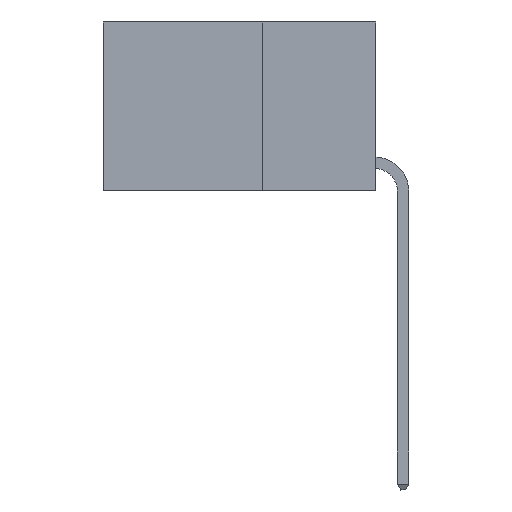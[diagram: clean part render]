
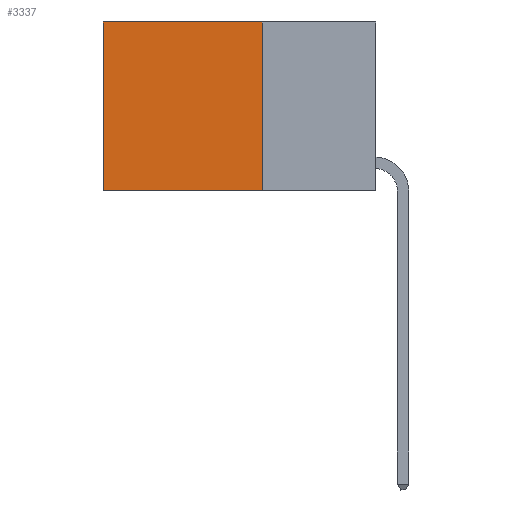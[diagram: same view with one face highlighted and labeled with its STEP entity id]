
A CAD part, left-side view. The second image highlights one B-rep face of the part: STEP entity #3337.
In plain terms, the highlighted planar face has unit normal (-1, 0, 0).
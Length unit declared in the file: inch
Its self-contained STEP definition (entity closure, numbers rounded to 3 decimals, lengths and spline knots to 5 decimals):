
#64 = CARTESIAN_POINT ( 'NONE',  ( 0.2625, 0.25, -0.37 ) ) ;
#413 = CARTESIAN_POINT ( 'NONE',  ( 0.2625, 0.6, 0. ) ) ;
#586 = CARTESIAN_POINT ( 'NONE',  ( 0.2625, 0.25, -0.37 ) ) ;
#1047 = AXIS2_PLACEMENT_3D ( 'NONE', #17012, #5316, #1689 ) ;
#1689 = DIRECTION ( 'NONE',  ( 0., 0., -1. ) ) ;
#3337 = ADVANCED_FACE ( 'NONE', ( #10134 ), #10241, .F. ) ;
#5316 = DIRECTION ( 'NONE',  ( 1., 0., 0. ) ) ;
#6028 = VECTOR ( 'NONE', #9191, 39.37008 ) ;
#6531 = VERTEX_POINT ( 'NONE', #8507 ) ;
#6735 = EDGE_CURVE ( 'NONE', #6531, #14203, #7397, .T. ) ;
#7397 = LINE ( 'NONE', #13955, #15891 ) ;
#8507 = CARTESIAN_POINT ( 'NONE',  ( 0.2625, 0.25, 0. ) ) ;
#8695 = ORIENTED_EDGE ( 'NONE', *, *, #10367, .T. ) ;
#9191 = DIRECTION ( 'NONE',  ( 0., 0., -1. ) ) ;
#9387 = VERTEX_POINT ( 'NONE', #586 ) ;
#9735 = LINE ( 'NONE', #11099, #17660 ) ;
#10134 = FACE_OUTER_BOUND ( 'NONE', #20794, .T. ) ;
#10232 = ORIENTED_EDGE ( 'NONE', *, *, #16934, .F. ) ;
#10241 = PLANE ( 'NONE',  #1047 ) ;
#10367 = EDGE_CURVE ( 'NONE', #14203, #20745, #9735, .T. ) ;
#10880 = CARTESIAN_POINT ( 'NONE',  ( 0.2625, 0.25, 0. ) ) ;
#11099 = CARTESIAN_POINT ( 'NONE',  ( 0.2625, 0.6, 0. ) ) ;
#12153 = VECTOR ( 'NONE', #18830, 39.37008 ) ;
#13955 = CARTESIAN_POINT ( 'NONE',  ( 0.2625, 0.25, 0. ) ) ;
#14203 = VERTEX_POINT ( 'NONE', #413 ) ;
#15026 = LINE ( 'NONE', #64, #12153 ) ;
#15891 = VECTOR ( 'NONE', #20777, 39.37008 ) ;
#16583 = CARTESIAN_POINT ( 'NONE',  ( 0.2625, 0.6, -0.37 ) ) ;
#16612 = DIRECTION ( 'NONE',  ( 0., 0., -1. ) ) ;
#16655 = ORIENTED_EDGE ( 'NONE', *, *, #20489, .F. ) ;
#16934 = EDGE_CURVE ( 'NONE', #6531, #9387, #19540, .T. ) ;
#17012 = CARTESIAN_POINT ( 'NONE',  ( 0.2625, 0.25, 0. ) ) ;
#17660 = VECTOR ( 'NONE', #16612, 39.37008 ) ;
#18830 = DIRECTION ( 'NONE',  ( 0., 1., 0. ) ) ;
#19540 = LINE ( 'NONE', #10880, #6028 ) ;
#20489 = EDGE_CURVE ( 'NONE', #9387, #20745, #15026, .T. ) ;
#20745 = VERTEX_POINT ( 'NONE', #16583 ) ;
#20777 = DIRECTION ( 'NONE',  ( 0., 1., 0. ) ) ;
#20794 = EDGE_LOOP ( 'NONE', ( #8695, #16655, #10232, #21432 ) ) ;
#21432 = ORIENTED_EDGE ( 'NONE', *, *, #6735, .T. ) ;
